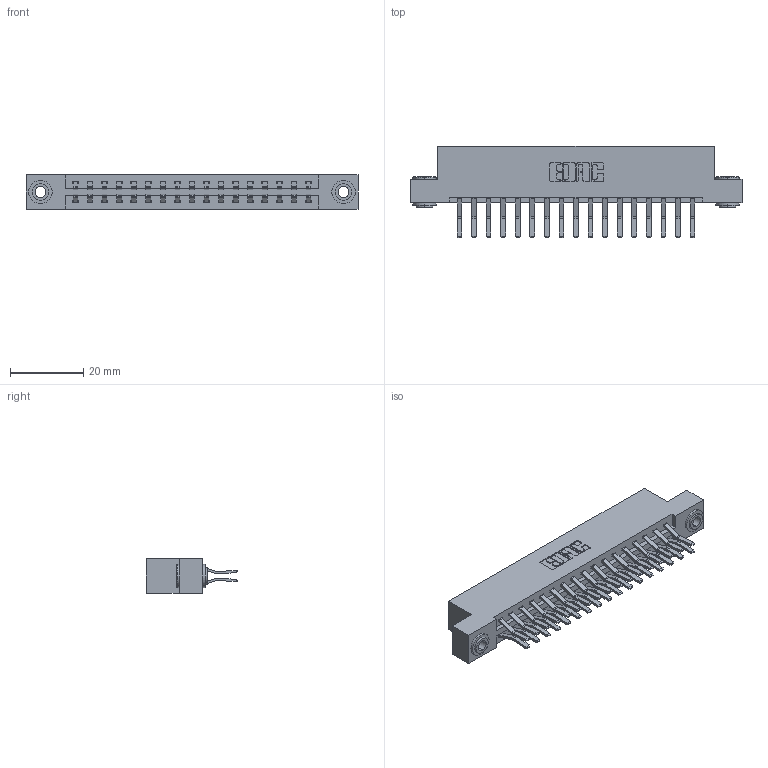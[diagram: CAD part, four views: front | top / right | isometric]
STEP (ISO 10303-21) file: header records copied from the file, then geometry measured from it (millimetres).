
FILE_DESCRIPTION (( 'STEP AP203' ), '1' );
FILE_NAME ('387-034-560-203.STEP', '2018-09-18T21:45:51', ( '' ), ( '' ), 'SwSTEP 2.0', 'SolidWorks 2016', '' );
FILE_SCHEMA (( 'CONFIG_CONTROL_DESIGN' ));
Length unit declared in the file: inch
Products named in the file (4): 345-292-001_560 Tail; 345-250-002_345-250-002-102; 387-034-560-203; 337 Part_Flush Mounting Lugs - 0.156 Dia-TH
Assembly tree (37 placements, depth 2):
  387-034-560-203
    337 Part_Flush Mounting Lugs - 0.156 Dia-TH
    345-292-001_560 Tail  x34
    345-250-002_345-250-002-102  x2
Bounding box: 90.37 x 24.78 x 9.4 mm (x, y, z)
Volume: 9433.7 mm3; surface area: 11291.4 mm2
Topology: 37 solids, 37 shells, 2056 faces, 6065 edges, 3994 vertices
Faces by surface type: plane 1372, cylinder 676, cone 8
Entity records: 17152 total; most frequent: CARTESIAN_POINT 2885, ORIENTED_EDGE 2814, DIRECTION 2537, EDGE_CURVE 1407, LINE 1251, VECTOR 1251, VERTEX_POINT 934, AXIS2_PLACEMENT_3D 643
